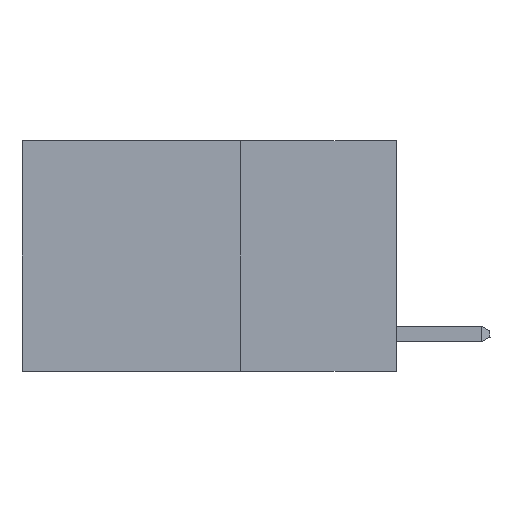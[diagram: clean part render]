
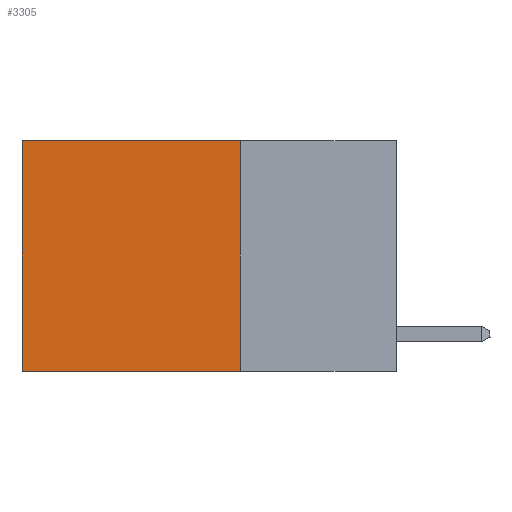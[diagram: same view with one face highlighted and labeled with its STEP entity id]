
A CAD part, left-side view. The second image highlights one B-rep face of the part: STEP entity #3305.
In plain terms, the highlighted planar face has unit normal (-1, 0, 0).
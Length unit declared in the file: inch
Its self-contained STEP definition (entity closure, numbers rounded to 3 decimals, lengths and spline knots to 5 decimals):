
#2074 = EDGE_LOOP ( 'NONE', ( #13371, #8423, #12008, #9125 ) ) ;
#2127 = VECTOR ( 'NONE', #9721, 39.37008 ) ;
#2619 = EDGE_CURVE ( 'NONE', #15890, #6393, #7562, .T. ) ;
#3305 = ADVANCED_FACE ( 'NONE', ( #13233 ), #7211, .F. ) ;
#3506 = CARTESIAN_POINT ( 'NONE',  ( 0.2625, 0.25, 0. ) ) ;
#4227 = VECTOR ( 'NONE', #21341, 39.37008 ) ;
#4385 = VERTEX_POINT ( 'NONE', #11335 ) ;
#5524 = CARTESIAN_POINT ( 'NONE',  ( 0.2625, 0.25, 0. ) ) ;
#5526 = LINE ( 'NONE', #13510, #2127 ) ;
#5728 = DIRECTION ( 'NONE',  ( 0., 0., -1. ) ) ;
#6393 = VERTEX_POINT ( 'NONE', #18204 ) ;
#7031 = EDGE_CURVE ( 'NONE', #10697, #4385, #19246, .T. ) ;
#7078 = DIRECTION ( 'NONE',  ( 0., 0., -1. ) ) ;
#7211 = PLANE ( 'NONE',  #12262 ) ;
#7562 = LINE ( 'NONE', #21267, #16312 ) ;
#8423 = ORIENTED_EDGE ( 'NONE', *, *, #19037, .F. ) ;
#9125 = ORIENTED_EDGE ( 'NONE', *, *, #13300, .T. ) ;
#9721 = DIRECTION ( 'NONE',  ( 0., 1., 0. ) ) ;
#10697 = VERTEX_POINT ( 'NONE', #3506 ) ;
#11010 = DIRECTION ( 'NONE',  ( 1., 0., 0. ) ) ;
#11335 = CARTESIAN_POINT ( 'NONE',  ( 0.2625, 0.25, -0.37 ) ) ;
#12008 = ORIENTED_EDGE ( 'NONE', *, *, #7031, .F. ) ;
#12262 = AXIS2_PLACEMENT_3D ( 'NONE', #16870, #11010, #7078 ) ;
#13233 = FACE_OUTER_BOUND ( 'NONE', #2074, .T. ) ;
#13248 = DIRECTION ( 'NONE',  ( 0., 0., -1. ) ) ;
#13300 = EDGE_CURVE ( 'NONE', #10697, #15890, #5526, .T. ) ;
#13371 = ORIENTED_EDGE ( 'NONE', *, *, #2619, .T. ) ;
#13510 = CARTESIAN_POINT ( 'NONE',  ( 0.2625, 0.25, 0. ) ) ;
#15890 = VERTEX_POINT ( 'NONE', #24630 ) ;
#16312 = VECTOR ( 'NONE', #5728, 39.37008 ) ;
#16870 = CARTESIAN_POINT ( 'NONE',  ( 0.2625, 0.25, 0. ) ) ;
#16902 = CARTESIAN_POINT ( 'NONE',  ( 0.2625, 0.25, -0.37 ) ) ;
#17032 = LINE ( 'NONE', #16902, #4227 ) ;
#18204 = CARTESIAN_POINT ( 'NONE',  ( 0.2625, 0.6, -0.37 ) ) ;
#19037 = EDGE_CURVE ( 'NONE', #4385, #6393, #17032, .T. ) ;
#19246 = LINE ( 'NONE', #5524, #20802 ) ;
#20802 = VECTOR ( 'NONE', #13248, 39.37008 ) ;
#21267 = CARTESIAN_POINT ( 'NONE',  ( 0.2625, 0.6, 0. ) ) ;
#21341 = DIRECTION ( 'NONE',  ( 0., 1., 0. ) ) ;
#24630 = CARTESIAN_POINT ( 'NONE',  ( 0.2625, 0.6, 0. ) ) ;
